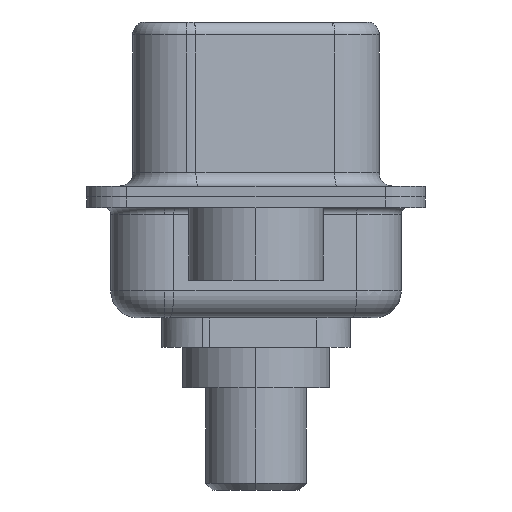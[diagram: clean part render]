
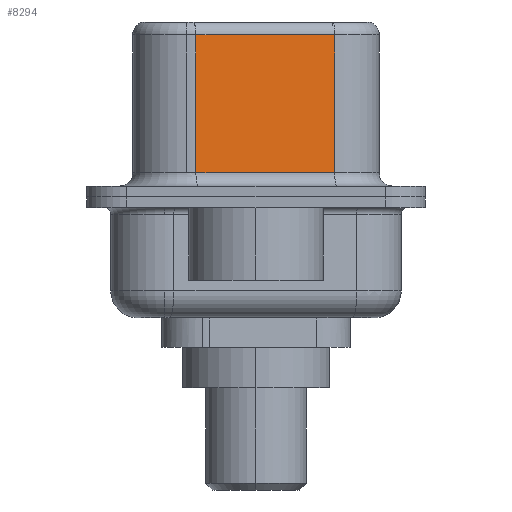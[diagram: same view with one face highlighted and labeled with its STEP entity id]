
A CAD part, left-side view. The second image highlights one B-rep face of the part: STEP entity #8294.
In plain terms, the highlighted planar face has unit normal (-0.985, -0.174, 0).
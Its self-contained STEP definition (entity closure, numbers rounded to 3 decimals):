
#682 = PLANE ( 'NONE',  #4765 ) ;
#1081 = DIRECTION ( 'NONE',  ( 0., 0., -1. ) ) ;
#1416 = VERTEX_POINT ( 'NONE', #13133 ) ;
#1652 = VECTOR ( 'NONE', #4999, 1000. ) ;
#1704 = EDGE_CURVE ( 'NONE', #2762, #8476, #5511, .T. ) ;
#1828 = VECTOR ( 'NONE', #1081, 1000. ) ;
#2354 = DIRECTION ( 'NONE',  ( -0.174, 0.985, 0. ) ) ;
#2608 = ORIENTED_EDGE ( 'NONE', *, *, #1704, .T. ) ;
#2762 = VERTEX_POINT ( 'NONE', #6431 ) ;
#3132 = DIRECTION ( 'NONE',  ( 0., 0., -1. ) ) ;
#3239 = ORIENTED_EDGE ( 'NONE', *, *, #16431, .T. ) ;
#3646 = VERTEX_POINT ( 'NONE', #8339 ) ;
#3980 = LINE ( 'NONE', #15531, #6509 ) ;
#4408 = CARTESIAN_POINT ( 'NONE',  ( 4.58, -2.927, 6.52 ) ) ;
#4765 = AXIS2_PLACEMENT_3D ( 'NONE', #11013, #12462, #15336 ) ;
#4999 = DIRECTION ( 'NONE',  ( 0.174, -0.985, 0. ) ) ;
#5511 = LINE ( 'NONE', #10788, #1652 ) ;
#6431 = CARTESIAN_POINT ( 'NONE',  ( 3.67, 2.233, 0.9 ) ) ;
#6509 = VECTOR ( 'NONE', #2354, 1000. ) ;
#8294 = ADVANCED_FACE ( 'NONE', ( #9732 ), #682, .F. ) ;
#8339 = CARTESIAN_POINT ( 'NONE',  ( 4.58, -2.927, 6.02 ) ) ;
#8431 = LINE ( 'NONE', #18665, #1828 ) ;
#8476 = VERTEX_POINT ( 'NONE', #10498 ) ;
#8695 = EDGE_CURVE ( 'NONE', #3646, #8476, #12904, .T. ) ;
#9732 = FACE_OUTER_BOUND ( 'NONE', #15331, .T. ) ;
#9810 = EDGE_CURVE ( 'NONE', #3646, #1416, #3980, .T. ) ;
#10498 = CARTESIAN_POINT ( 'NONE',  ( 4.58, -2.927, 0.9 ) ) ;
#10788 = CARTESIAN_POINT ( 'NONE',  ( 4.58, -2.927, 0.9 ) ) ;
#11013 = CARTESIAN_POINT ( 'NONE',  ( 4.58, -2.927, 6.52 ) ) ;
#12462 = DIRECTION ( 'NONE',  ( 0.985, 0.174, 0. ) ) ;
#12575 = ORIENTED_EDGE ( 'NONE', *, *, #8695, .F. ) ;
#12904 = LINE ( 'NONE', #4408, #15656 ) ;
#13094 = ORIENTED_EDGE ( 'NONE', *, *, #9810, .T. ) ;
#13133 = CARTESIAN_POINT ( 'NONE',  ( 3.67, 2.233, 6.02 ) ) ;
#15331 = EDGE_LOOP ( 'NONE', ( #12575, #13094, #3239, #2608 ) ) ;
#15336 = DIRECTION ( 'NONE',  ( -0.174, 0.985, 0. ) ) ;
#15531 = CARTESIAN_POINT ( 'NONE',  ( 4.58, -2.927, 6.02 ) ) ;
#15656 = VECTOR ( 'NONE', #3132, 1000. ) ;
#16431 = EDGE_CURVE ( 'NONE', #1416, #2762, #8431, .T. ) ;
#18665 = CARTESIAN_POINT ( 'NONE',  ( 3.67, 2.233, 6.52 ) ) ;
